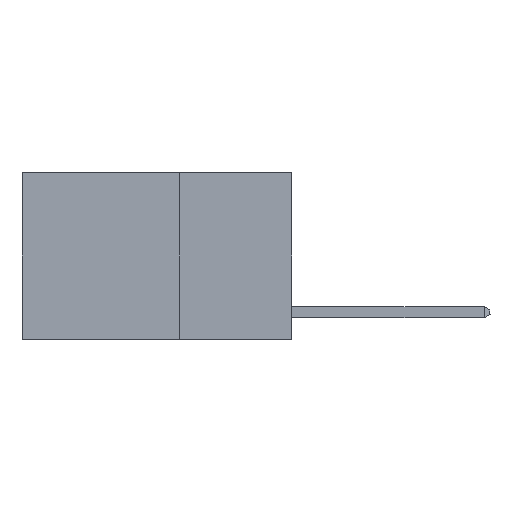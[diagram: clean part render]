
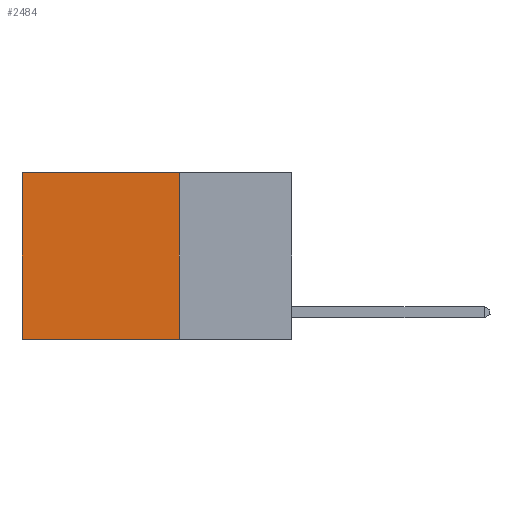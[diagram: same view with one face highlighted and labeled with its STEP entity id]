
A CAD part, left-side view. The second image highlights one B-rep face of the part: STEP entity #2484.
In plain terms, the highlighted planar face has unit normal (-1, 0, 0).
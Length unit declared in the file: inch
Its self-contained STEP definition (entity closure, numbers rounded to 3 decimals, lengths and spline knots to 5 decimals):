
#624 = EDGE_CURVE ( 'NONE', #12989, #5622, #5767, .T. ) ;
#776 = DIRECTION ( 'NONE',  ( 0., 0., -1. ) ) ;
#811 = ORIENTED_EDGE ( 'NONE', *, *, #624, .T. ) ;
#1097 = CARTESIAN_POINT ( 'NONE',  ( 0.2625, 0.25, 0. ) ) ;
#1243 = LINE ( 'NONE', #13138, #8081 ) ;
#2028 = LINE ( 'NONE', #10600, #8501 ) ;
#2259 = DIRECTION ( 'NONE',  ( 0., 0., -1. ) ) ;
#2484 = ADVANCED_FACE ( 'NONE', ( #6442 ), #3776, .F. ) ;
#2572 = VECTOR ( 'NONE', #14182, 39.37008 ) ;
#2600 = EDGE_LOOP ( 'NONE', ( #15573, #12908, #6375, #811 ) ) ;
#3256 = EDGE_CURVE ( 'NONE', #5622, #8158, #1243, .T. ) ;
#3487 = AXIS2_PLACEMENT_3D ( 'NONE', #14709, #6219, #11155 ) ;
#3776 = PLANE ( 'NONE',  #3487 ) ;
#5622 = VERTEX_POINT ( 'NONE', #8426 ) ;
#5760 = CARTESIAN_POINT ( 'NONE',  ( 0.2625, 0.25, -0.37 ) ) ;
#5767 = LINE ( 'NONE', #6872, #2572 ) ;
#6219 = DIRECTION ( 'NONE',  ( 1., 0., 0. ) ) ;
#6375 = ORIENTED_EDGE ( 'NONE', *, *, #7614, .F. ) ;
#6442 = FACE_OUTER_BOUND ( 'NONE', #2600, .T. ) ;
#6872 = CARTESIAN_POINT ( 'NONE',  ( 0.2625, 0.25, 0. ) ) ;
#7196 = VECTOR ( 'NONE', #12852, 39.37008 ) ;
#7339 = EDGE_CURVE ( 'NONE', #15337, #8158, #8017, .T. ) ;
#7546 = CARTESIAN_POINT ( 'NONE',  ( 0.2625, 0.25, -0.37 ) ) ;
#7614 = EDGE_CURVE ( 'NONE', #12989, #15337, #2028, .T. ) ;
#8017 = LINE ( 'NONE', #5760, #7196 ) ;
#8081 = VECTOR ( 'NONE', #2259, 39.37008 ) ;
#8158 = VERTEX_POINT ( 'NONE', #13716 ) ;
#8426 = CARTESIAN_POINT ( 'NONE',  ( 0.2625, 0.6, 0. ) ) ;
#8501 = VECTOR ( 'NONE', #776, 39.37008 ) ;
#10600 = CARTESIAN_POINT ( 'NONE',  ( 0.2625, 0.25, 0. ) ) ;
#11155 = DIRECTION ( 'NONE',  ( 0., 0., -1. ) ) ;
#12852 = DIRECTION ( 'NONE',  ( 0., 1., 0. ) ) ;
#12908 = ORIENTED_EDGE ( 'NONE', *, *, #7339, .F. ) ;
#12989 = VERTEX_POINT ( 'NONE', #1097 ) ;
#13138 = CARTESIAN_POINT ( 'NONE',  ( 0.2625, 0.6, 0. ) ) ;
#13716 = CARTESIAN_POINT ( 'NONE',  ( 0.2625, 0.6, -0.37 ) ) ;
#14182 = DIRECTION ( 'NONE',  ( 0., 1., 0. ) ) ;
#14709 = CARTESIAN_POINT ( 'NONE',  ( 0.2625, 0.25, 0. ) ) ;
#15337 = VERTEX_POINT ( 'NONE', #7546 ) ;
#15573 = ORIENTED_EDGE ( 'NONE', *, *, #3256, .T. ) ;
